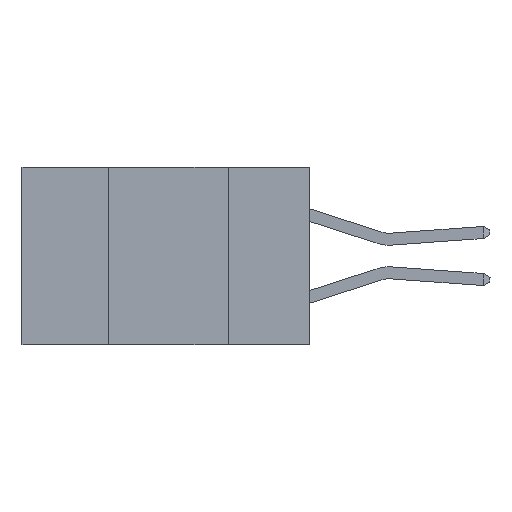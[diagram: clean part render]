
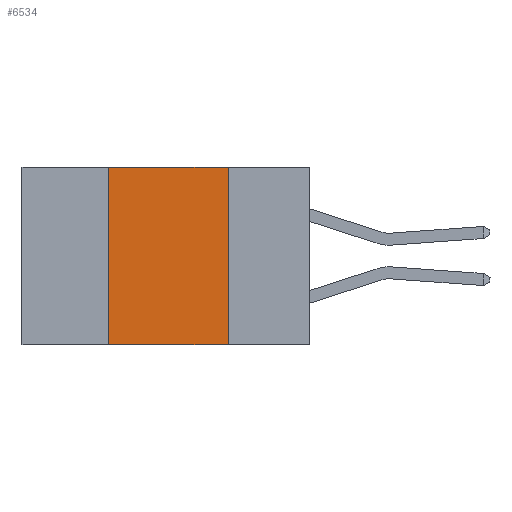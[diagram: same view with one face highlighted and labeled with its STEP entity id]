
A CAD part, left-side view. The second image highlights one B-rep face of the part: STEP entity #6534.
In plain terms, the highlighted planar face has unit normal (-1, 0, 0).
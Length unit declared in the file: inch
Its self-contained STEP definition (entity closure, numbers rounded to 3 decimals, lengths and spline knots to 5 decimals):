
#506 = VECTOR ( 'NONE', #1728, 39.37008 ) ;
#582 = CARTESIAN_POINT ( 'NONE',  ( 0., 0.6, 0. ) ) ;
#1047 = ORIENTED_EDGE ( 'NONE', *, *, #18108, .F. ) ;
#1369 = EDGE_CURVE ( 'NONE', #23714, #14754, #15236, .T. ) ;
#1728 = DIRECTION ( 'NONE',  ( 0., 0., 1. ) ) ;
#4363 = CARTESIAN_POINT ( 'NONE',  ( 0., 0.17, -0.37 ) ) ;
#5166 = AXIS2_PLACEMENT_3D ( 'NONE', #23252, #23119, #23102 ) ;
#5278 = LINE ( 'NONE', #582, #19404 ) ;
#6071 = DIRECTION ( 'NONE',  ( 0., -1., 0. ) ) ;
#6534 = ADVANCED_FACE ( 'NONE', ( #23628 ), #23125, .F. ) ;
#7605 = ORIENTED_EDGE ( 'NONE', *, *, #21136, .F. ) ;
#7844 = VECTOR ( 'NONE', #10303, 39.37008 ) ;
#7941 = CARTESIAN_POINT ( 'NONE',  ( 0., 0.6, -0.37 ) ) ;
#10209 = DIRECTION ( 'NONE',  ( 0., -1., 0. ) ) ;
#10215 = CARTESIAN_POINT ( 'NONE',  ( 0., 0.17, -0.37 ) ) ;
#10303 = DIRECTION ( 'NONE',  ( 0., 0., -1. ) ) ;
#10367 = EDGE_LOOP ( 'NONE', ( #7605, #1047, #21698, #20706 ) ) ;
#11791 = LINE ( 'NONE', #7941, #16864 ) ;
#14405 = EDGE_CURVE ( 'NONE', #23714, #21090, #11791, .T. ) ;
#14754 = VERTEX_POINT ( 'NONE', #24128 ) ;
#15236 = LINE ( 'NONE', #21992, #506 ) ;
#16864 = VECTOR ( 'NONE', #6071, 39.37008 ) ;
#18108 = EDGE_CURVE ( 'NONE', #14754, #22100, #5278, .T. ) ;
#18274 = CARTESIAN_POINT ( 'NONE',  ( 0., 0.42, -0.37 ) ) ;
#19404 = VECTOR ( 'NONE', #10209, 39.37008 ) ;
#20706 = ORIENTED_EDGE ( 'NONE', *, *, #14405, .T. ) ;
#21090 = VERTEX_POINT ( 'NONE', #4363 ) ;
#21136 = EDGE_CURVE ( 'NONE', #22100, #21090, #23090, .T. ) ;
#21698 = ORIENTED_EDGE ( 'NONE', *, *, #1369, .F. ) ;
#21992 = CARTESIAN_POINT ( 'NONE',  ( 0., 0.42, -0.37 ) ) ;
#22100 = VERTEX_POINT ( 'NONE', #22981 ) ;
#22981 = CARTESIAN_POINT ( 'NONE',  ( 0., 0.17, 0. ) ) ;
#23090 = LINE ( 'NONE', #10215, #7844 ) ;
#23102 = DIRECTION ( 'NONE',  ( 0., 0., -1. ) ) ;
#23119 = DIRECTION ( 'NONE',  ( 1., 0., 0. ) ) ;
#23125 = PLANE ( 'NONE',  #5166 ) ;
#23252 = CARTESIAN_POINT ( 'NONE',  ( 0., 0.6, 0. ) ) ;
#23628 = FACE_OUTER_BOUND ( 'NONE', #10367, .T. ) ;
#23714 = VERTEX_POINT ( 'NONE', #18274 ) ;
#24128 = CARTESIAN_POINT ( 'NONE',  ( 0., 0.42, 0. ) ) ;
